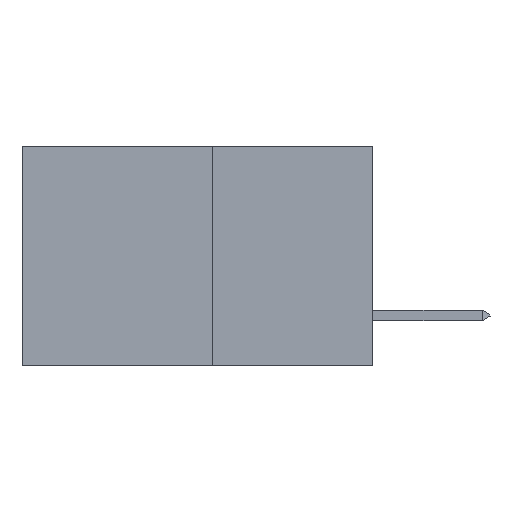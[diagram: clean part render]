
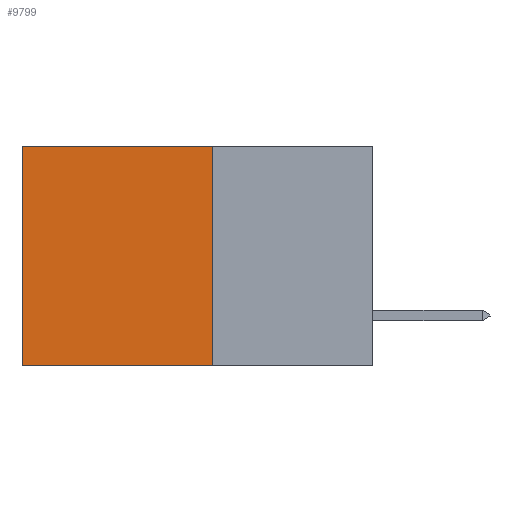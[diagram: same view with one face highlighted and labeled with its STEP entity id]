
A CAD part, left-side view. The second image highlights one B-rep face of the part: STEP entity #9799.
In plain terms, the highlighted planar face has unit normal (-1, 0, 0).
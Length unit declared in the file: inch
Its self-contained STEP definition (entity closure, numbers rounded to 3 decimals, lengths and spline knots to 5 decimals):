
#109 = DIRECTION ( 'NONE',  ( 0., 0., -1. ) ) ;
#263 = PLANE ( 'NONE',  #12919 ) ;
#982 = EDGE_LOOP ( 'NONE', ( #3942, #3528, #2901, #8847 ) ) ;
#1576 = EDGE_CURVE ( 'NONE', #4901, #7155, #7297, .T. ) ;
#2061 = VERTEX_POINT ( 'NONE', #6887 ) ;
#2641 = DIRECTION ( 'NONE',  ( 0., 0., -1. ) ) ;
#2901 = ORIENTED_EDGE ( 'NONE', *, *, #7938, .F. ) ;
#2918 = CARTESIAN_POINT ( 'NONE',  ( 0.277, 0.27, 0. ) ) ;
#3419 = VECTOR ( 'NONE', #3483, 39.37008 ) ;
#3483 = DIRECTION ( 'NONE',  ( 0., 0., -1. ) ) ;
#3528 = ORIENTED_EDGE ( 'NONE', *, *, #1576, .F. ) ;
#3713 = CARTESIAN_POINT ( 'NONE',  ( 0.277, 0.27, -0.37 ) ) ;
#3775 = EDGE_CURVE ( 'NONE', #7603, #2061, #13421, .T. ) ;
#3942 = ORIENTED_EDGE ( 'NONE', *, *, #12670, .T. ) ;
#4090 = DIRECTION ( 'NONE',  ( 0., 1., 0. ) ) ;
#4634 = CARTESIAN_POINT ( 'NONE',  ( 0.277, 0.59, -0.37 ) ) ;
#4901 = VERTEX_POINT ( 'NONE', #11260 ) ;
#5341 = VECTOR ( 'NONE', #4090, 39.37008 ) ;
#6887 = CARTESIAN_POINT ( 'NONE',  ( 0.277, 0.59, 0. ) ) ;
#7155 = VERTEX_POINT ( 'NONE', #4634 ) ;
#7219 = CARTESIAN_POINT ( 'NONE',  ( 0.277, 0.27, -0.37 ) ) ;
#7297 = LINE ( 'NONE', #7219, #12848 ) ;
#7603 = VERTEX_POINT ( 'NONE', #10706 ) ;
#7938 = EDGE_CURVE ( 'NONE', #7603, #4901, #13927, .T. ) ;
#8751 = VECTOR ( 'NONE', #109, 39.37008 ) ;
#8847 = ORIENTED_EDGE ( 'NONE', *, *, #3775, .T. ) ;
#9281 = LINE ( 'NONE', #9990, #3419 ) ;
#9315 = DIRECTION ( 'NONE',  ( 1., 0., 0. ) ) ;
#9799 = ADVANCED_FACE ( 'NONE', ( #12528 ), #263, .F. ) ;
#9990 = CARTESIAN_POINT ( 'NONE',  ( 0.277, 0.59, -0.37 ) ) ;
#10706 = CARTESIAN_POINT ( 'NONE',  ( 0.277, 0.27, 0. ) ) ;
#11260 = CARTESIAN_POINT ( 'NONE',  ( 0.277, 0.27, -0.37 ) ) ;
#12528 = FACE_OUTER_BOUND ( 'NONE', #982, .T. ) ;
#12670 = EDGE_CURVE ( 'NONE', #2061, #7155, #9281, .T. ) ;
#12848 = VECTOR ( 'NONE', #13545, 39.37008 ) ;
#12919 = AXIS2_PLACEMENT_3D ( 'NONE', #13442, #9315, #2641 ) ;
#13421 = LINE ( 'NONE', #2918, #5341 ) ;
#13442 = CARTESIAN_POINT ( 'NONE',  ( 0.277, 0.27, -0.37 ) ) ;
#13545 = DIRECTION ( 'NONE',  ( 0., 1., 0. ) ) ;
#13927 = LINE ( 'NONE', #3713, #8751 ) ;
